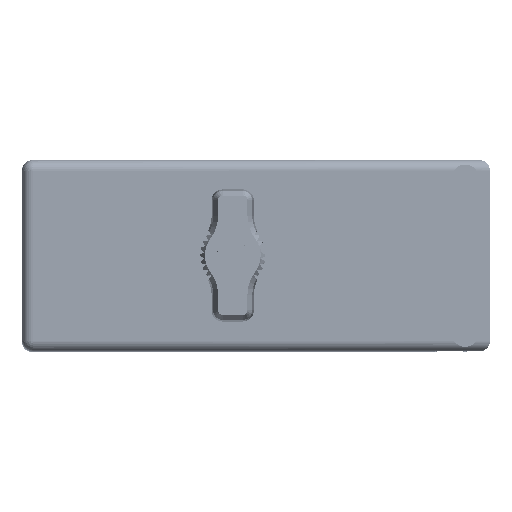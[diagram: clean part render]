
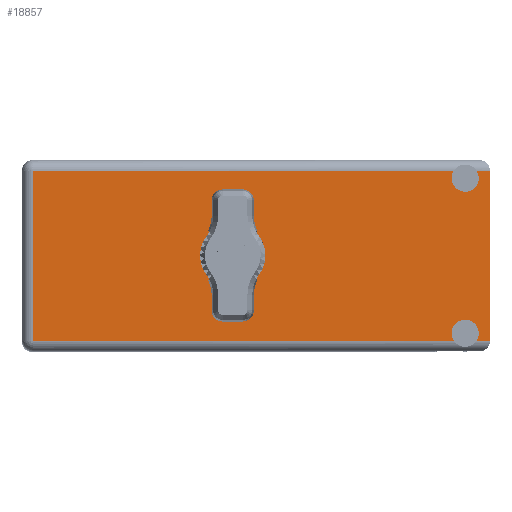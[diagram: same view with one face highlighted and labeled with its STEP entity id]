
A CAD part, top view. The second image highlights one B-rep face of the part: STEP entity #18857.
In plain terms, the highlighted face is planar.
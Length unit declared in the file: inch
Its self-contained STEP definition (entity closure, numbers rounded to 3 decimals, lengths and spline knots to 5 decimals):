
#1536 = CARTESIAN_POINT ( 'NONE',  ( 2.78419, 1.775, -1.164 ) ) ;
#2035 = DIRECTION ( 'NONE',  ( 0., 1., 0. ) ) ;
#2322 = CARTESIAN_POINT ( 'NONE',  ( 2.858, 1.775, -0.117 ) ) ;
#3696 = VECTOR ( 'NONE', #69250, 39.37008 ) ;
#3706 = EDGE_CURVE ( 'NONE', #78413, #78480, #83927, .T. ) ;
#4129 = DIRECTION ( 'NONE',  ( 0., 0., 1. ) ) ;
#5153 = CARTESIAN_POINT ( 'NONE',  ( 0.07, 1.775, -0.07 ) ) ;
#6117 = VECTOR ( 'NONE', #56535, 39.37008 ) ;
#6446 = CIRCLE ( 'NONE', #13767, 0.0875 ) ;
#8556 = DIRECTION ( 'NONE',  ( 0., 1., 0. ) ) ;
#9362 = CARTESIAN_POINT ( 'NONE',  ( 2.93181, 1.775, -1.164 ) ) ;
#10182 = ORIENTED_EDGE ( 'NONE', *, *, #36201, .F. ) ;
#12361 = CIRCLE ( 'NONE', #64339, 0.0875 ) ;
#13767 = AXIS2_PLACEMENT_3D ( 'NONE', #86413, #17407, #4129 ) ;
#14052 = AXIS2_PLACEMENT_3D ( 'NONE', #33756, #26194, #33153 ) ;
#15899 = DIRECTION ( 'NONE',  ( -1., 0., 0. ) ) ;
#16414 = AXIS2_PLACEMENT_3D ( 'NONE', #49887, #8556, #56534 ) ;
#17407 = DIRECTION ( 'NONE',  ( 0., 1., 0. ) ) ;
#18191 = VECTOR ( 'NONE', #65760, 39.37008 ) ;
#18857 = ADVANCED_FACE ( 'NONE', ( #47107, #25503 ), #19553, .T. ) ;
#19499 = CIRCLE ( 'NONE', #52460, 0.125 ) ;
#19553 = PLANE ( 'NONE',  #14052 ) ;
#19673 = VECTOR ( 'NONE', #15899, 39.37008 ) ;
#20547 = VERTEX_POINT ( 'NONE', #29815 ) ;
#20560 = CARTESIAN_POINT ( 'NONE',  ( 2.78419, 1.775, -0.07 ) ) ;
#21222 = ORIENTED_EDGE ( 'NONE', *, *, #75168, .F. ) ;
#22260 = LINE ( 'NONE', #43276, #6117 ) ;
#23990 = VERTEX_POINT ( 'NONE', #77612 ) ;
#24178 = EDGE_CURVE ( 'NONE', #52165, #78413, #27942, .T. ) ;
#25503 = FACE_OUTER_BOUND ( 'NONE', #37946, .T. ) ;
#26194 = DIRECTION ( 'NONE',  ( 0., 1., 0. ) ) ;
#26281 = CIRCLE ( 'NONE', #16414, 0.0875 ) ;
#26378 = AXIS2_PLACEMENT_3D ( 'NONE', #69365, #48239, #34974 ) ;
#27942 = LINE ( 'NONE', #78200, #70038 ) ;
#29526 = ORIENTED_EDGE ( 'NONE', *, *, #60647, .T. ) ;
#29786 = CARTESIAN_POINT ( 'NONE',  ( 0., 1.775, -1.164 ) ) ;
#29815 = CARTESIAN_POINT ( 'NONE',  ( 2.93181, 1.775, -0.07 ) ) ;
#30219 = VERTEX_POINT ( 'NONE', #9362 ) ;
#31105 = CARTESIAN_POINT ( 'NONE',  ( 1.359, 1.775, -0.742 ) ) ;
#32439 = CARTESIAN_POINT ( 'NONE',  ( 2.858, 1.775, -0.2045 ) ) ;
#32448 = ORIENTED_EDGE ( 'NONE', *, *, #70325, .F. ) ;
#33153 = DIRECTION ( 'NONE',  ( 0., 0., 1. ) ) ;
#33351 = ORIENTED_EDGE ( 'NONE', *, *, #84348, .T. ) ;
#33756 = CARTESIAN_POINT ( 'NONE',  ( 0., 1.775, -1.234 ) ) ;
#34974 = DIRECTION ( 'NONE',  ( 0., 0., 1. ) ) ;
#35207 = VERTEX_POINT ( 'NONE', #53110 ) ;
#35730 = ORIENTED_EDGE ( 'NONE', *, *, #24178, .T. ) ;
#36053 = CARTESIAN_POINT ( 'NONE',  ( 0.07, 1.775, -1.234 ) ) ;
#36201 = EDGE_CURVE ( 'NONE', #35207, #78178, #41551, .T. ) ;
#37946 = EDGE_LOOP ( 'NONE', ( #48329, #21222, #74733, #29526, #10182, #33351, #51034, #32448, #35730, #87518 ) ) ;
#41551 = LINE ( 'NONE', #76424, #3696 ) ;
#43185 = VERTEX_POINT ( 'NONE', #32439 ) ;
#43276 = CARTESIAN_POINT ( 'NONE',  ( 3.018, 1.775, -0.07 ) ) ;
#45888 = CARTESIAN_POINT ( 'NONE',  ( 3.018, 1.775, -0.07 ) ) ;
#47107 = FACE_BOUND ( 'NONE', #53578, .T. ) ;
#48239 = DIRECTION ( 'NONE',  ( 0., 1., 0. ) ) ;
#48312 = DIRECTION ( 'NONE',  ( 0., 1., 0. ) ) ;
#48329 = ORIENTED_EDGE ( 'NONE', *, *, #86851, .T. ) ;
#49222 = ORIENTED_EDGE ( 'NONE', *, *, #69902, .F. ) ;
#49278 = CARTESIAN_POINT ( 'NONE',  ( 1.359, 1.775, -0.617 ) ) ;
#49817 = VERTEX_POINT ( 'NONE', #20560 ) ;
#49887 = CARTESIAN_POINT ( 'NONE',  ( 2.858, 1.775, -0.117 ) ) ;
#51034 = ORIENTED_EDGE ( 'NONE', *, *, #54900, .F. ) ;
#52165 = VERTEX_POINT ( 'NONE', #1536 ) ;
#52460 = AXIS2_PLACEMENT_3D ( 'NONE', #49278, #84480, #77866 ) ;
#53110 = CARTESIAN_POINT ( 'NONE',  ( 3.018, 1.775, -1.164 ) ) ;
#53578 = EDGE_LOOP ( 'NONE', ( #49222, #78241 ) ) ;
#53781 = LINE ( 'NONE', #45888, #18191 ) ;
#54383 = CARTESIAN_POINT ( 'NONE',  ( 2.858, 1.775, -1.117 ) ) ;
#54900 = EDGE_CURVE ( 'NONE', #78659, #30219, #69537, .T. ) ;
#56534 = DIRECTION ( 'NONE',  ( 0., 0., 1. ) ) ;
#56535 = DIRECTION ( 'NONE',  ( 1., 0., 0. ) ) ;
#60647 = EDGE_CURVE ( 'NONE', #20547, #78178, #22260, .T. ) ;
#60654 = CARTESIAN_POINT ( 'NONE',  ( 0.07, 1.775, -1.164 ) ) ;
#62104 = VERTEX_POINT ( 'NONE', #31105 ) ;
#63434 = VECTOR ( 'NONE', #70152, 39.37008 ) ;
#64327 = DIRECTION ( 'NONE',  ( -1., 0., 0. ) ) ;
#64339 = AXIS2_PLACEMENT_3D ( 'NONE', #2322, #2035, #70523 ) ;
#65169 = CIRCLE ( 'NONE', #26378, 0.125 ) ;
#65760 = DIRECTION ( 'NONE',  ( 1., 0., 0. ) ) ;
#66341 = EDGE_CURVE ( 'NONE', #62104, #23990, #65169, .T. ) ;
#67937 = DIRECTION ( 'NONE',  ( 0., 0., 1. ) ) ;
#69250 = DIRECTION ( 'NONE',  ( 0., 0., 1. ) ) ;
#69274 = LINE ( 'NONE', #29786, #19673 ) ;
#69365 = CARTESIAN_POINT ( 'NONE',  ( 1.359, 1.775, -0.617 ) ) ;
#69537 = CIRCLE ( 'NONE', #74881, 0.0875 ) ;
#69902 = EDGE_CURVE ( 'NONE', #23990, #62104, #19499, .T. ) ;
#70038 = VECTOR ( 'NONE', #64327, 39.37008 ) ;
#70152 = DIRECTION ( 'NONE',  ( 0., 0., 1. ) ) ;
#70325 = EDGE_CURVE ( 'NONE', #52165, #78659, #6446, .T. ) ;
#70523 = DIRECTION ( 'NONE',  ( 0., 0., 1. ) ) ;
#70853 = CARTESIAN_POINT ( 'NONE',  ( 2.858, 1.775, -1.0295 ) ) ;
#74547 = EDGE_CURVE ( 'NONE', #20547, #43185, #12361, .T. ) ;
#74733 = ORIENTED_EDGE ( 'NONE', *, *, #74547, .F. ) ;
#74881 = AXIS2_PLACEMENT_3D ( 'NONE', #54383, #48312, #67937 ) ;
#75168 = EDGE_CURVE ( 'NONE', #43185, #49817, #26281, .T. ) ;
#76424 = CARTESIAN_POINT ( 'NONE',  ( 3.018, 1.775, 0. ) ) ;
#77612 = CARTESIAN_POINT ( 'NONE',  ( 1.359, 1.775, -0.492 ) ) ;
#77866 = DIRECTION ( 'NONE',  ( 0., 0., 1. ) ) ;
#78178 = VERTEX_POINT ( 'NONE', #78443 ) ;
#78200 = CARTESIAN_POINT ( 'NONE',  ( 0., 1.775, -1.164 ) ) ;
#78241 = ORIENTED_EDGE ( 'NONE', *, *, #66341, .F. ) ;
#78413 = VERTEX_POINT ( 'NONE', #60654 ) ;
#78443 = CARTESIAN_POINT ( 'NONE',  ( 3.018, 1.775, -0.07 ) ) ;
#78480 = VERTEX_POINT ( 'NONE', #5153 ) ;
#78659 = VERTEX_POINT ( 'NONE', #70853 ) ;
#83927 = LINE ( 'NONE', #36053, #63434 ) ;
#84348 = EDGE_CURVE ( 'NONE', #35207, #30219, #69274, .T. ) ;
#84480 = DIRECTION ( 'NONE',  ( 0., 1., 0. ) ) ;
#86413 = CARTESIAN_POINT ( 'NONE',  ( 2.858, 1.775, -1.117 ) ) ;
#86851 = EDGE_CURVE ( 'NONE', #78480, #49817, #53781, .T. ) ;
#87518 = ORIENTED_EDGE ( 'NONE', *, *, #3706, .T. ) ;
